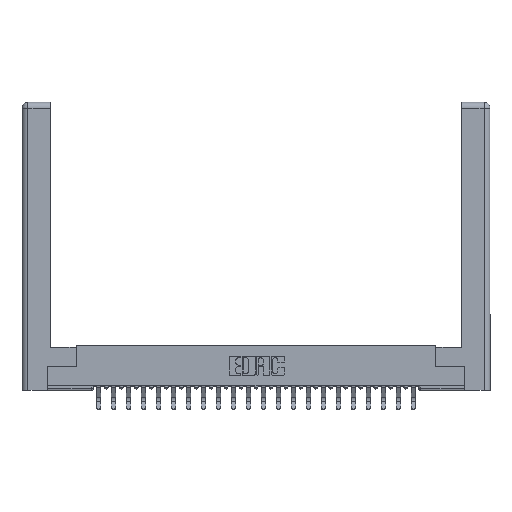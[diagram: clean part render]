
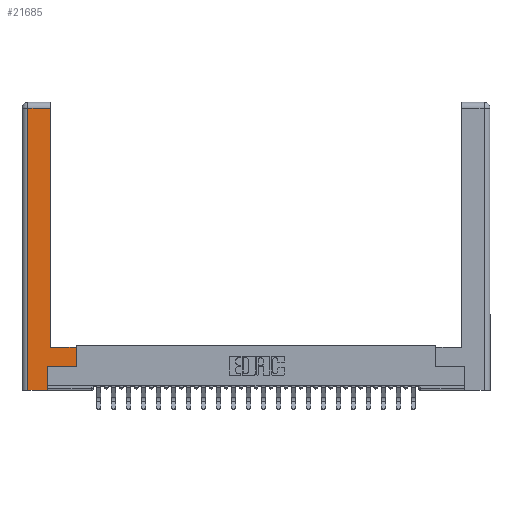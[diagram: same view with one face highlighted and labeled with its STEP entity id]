
A CAD part, top view. The second image highlights one B-rep face of the part: STEP entity #21685.
In plain terms, the highlighted planar face has unit normal (0, 0, 1).
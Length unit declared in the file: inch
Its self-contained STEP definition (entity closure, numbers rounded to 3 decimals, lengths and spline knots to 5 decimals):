
#400 = LINE ( 'NONE', #23113, #10214 ) ;
#420 = CARTESIAN_POINT ( 'NONE',  ( 0.295, 3., 0. ) ) ;
#613 = EDGE_CURVE ( 'NONE', #2396, #14917, #5931, .T. ) ;
#748 = DIRECTION ( 'NONE',  ( -1., 0., 0. ) ) ;
#963 = EDGE_LOOP ( 'NONE', ( #10906, #6641, #12486, #24524, #22520, #22392, #9960, #10470 ) ) ;
#1073 = VECTOR ( 'NONE', #14749, 39.37008 ) ;
#1088 = DIRECTION ( 'NONE',  ( -1., 0., 0. ) ) ;
#1736 = VECTOR ( 'NONE', #748, 39.37008 ) ;
#2396 = VERTEX_POINT ( 'NONE', #5903 ) ;
#2397 = FACE_OUTER_BOUND ( 'NONE', #963, .T. ) ;
#2955 = CARTESIAN_POINT ( 'NONE',  ( 0.0615, 2.94, 0. ) ) ;
#3697 = CARTESIAN_POINT ( 'NONE',  ( 0.265, 0., 0. ) ) ;
#3788 = DIRECTION ( 'NONE',  ( 0., 1., 0. ) ) ;
#4663 = CARTESIAN_POINT ( 'NONE',  ( 0., 0., 0. ) ) ;
#5903 = CARTESIAN_POINT ( 'NONE',  ( 0.295, 0.45, 0. ) ) ;
#5931 = LINE ( 'NONE', #420, #24735 ) ;
#6381 = VERTEX_POINT ( 'NONE', #22027 ) ;
#6532 = DIRECTION ( 'NONE',  ( -1., 0., 0. ) ) ;
#6641 = ORIENTED_EDGE ( 'NONE', *, *, #16748, .T. ) ;
#6659 = CARTESIAN_POINT ( 'NONE',  ( 0.0615, 2.94, 0. ) ) ;
#6730 = CARTESIAN_POINT ( 'NONE',  ( 0.295, 2.94, 0. ) ) ;
#7109 = CARTESIAN_POINT ( 'NONE',  ( 0.565, 0.45, 0. ) ) ;
#7925 = DIRECTION ( 'NONE',  ( 0., -1., 0. ) ) ;
#8385 = AXIS2_PLACEMENT_3D ( 'NONE', #4663, #23725, #6532 ) ;
#8947 = VECTOR ( 'NONE', #18878, 39.37008 ) ;
#9960 = ORIENTED_EDGE ( 'NONE', *, *, #19291, .T. ) ;
#10214 = VECTOR ( 'NONE', #13572, 39.37008 ) ;
#10261 = LINE ( 'NONE', #17926, #1736 ) ;
#10470 = ORIENTED_EDGE ( 'NONE', *, *, #11905, .T. ) ;
#10906 = ORIENTED_EDGE ( 'NONE', *, *, #613, .T. ) ;
#10980 = DIRECTION ( 'NONE',  ( 1., 0., 0. ) ) ;
#11434 = CARTESIAN_POINT ( 'NONE',  ( 0.565, 0.245, 0. ) ) ;
#11905 = EDGE_CURVE ( 'NONE', #16444, #2396, #10261, .T. ) ;
#12083 = VERTEX_POINT ( 'NONE', #3697 ) ;
#12486 = ORIENTED_EDGE ( 'NONE', *, *, #21591, .T. ) ;
#12866 = LINE ( 'NONE', #7109, #1073 ) ;
#13144 = LINE ( 'NONE', #20790, #8947 ) ;
#13359 = EDGE_CURVE ( 'NONE', #16351, #12083, #13144, .T. ) ;
#13572 = DIRECTION ( 'NONE',  ( 0., 1., 0. ) ) ;
#14389 = CARTESIAN_POINT ( 'NONE',  ( 0.565, 0.245, 0. ) ) ;
#14749 = DIRECTION ( 'NONE',  ( 0., 1., 0. ) ) ;
#14767 = VECTOR ( 'NONE', #7925, 39.37008 ) ;
#14917 = VERTEX_POINT ( 'NONE', #6730 ) ;
#16267 = LINE ( 'NONE', #2955, #17851 ) ;
#16351 = VERTEX_POINT ( 'NONE', #16780 ) ;
#16444 = VERTEX_POINT ( 'NONE', #17019 ) ;
#16748 = EDGE_CURVE ( 'NONE', #14917, #24480, #16267, .T. ) ;
#16780 = CARTESIAN_POINT ( 'NONE',  ( 0.0615, 0., 0. ) ) ;
#17019 = CARTESIAN_POINT ( 'NONE',  ( 0.565, 0.45, 0. ) ) ;
#17832 = PLANE ( 'NONE',  #8385 ) ;
#17851 = VECTOR ( 'NONE', #1088, 39.37008 ) ;
#17880 = EDGE_CURVE ( 'NONE', #6381, #24100, #24411, .T. ) ;
#17926 = CARTESIAN_POINT ( 'NONE',  ( 0.295, 0.45, 0. ) ) ;
#18831 = LINE ( 'NONE', #18943, #14767 ) ;
#18878 = DIRECTION ( 'NONE',  ( 1., 0., 0. ) ) ;
#18943 = CARTESIAN_POINT ( 'NONE',  ( 0.0615, 0., 0. ) ) ;
#19291 = EDGE_CURVE ( 'NONE', #24100, #16444, #12866, .T. ) ;
#20790 = CARTESIAN_POINT ( 'NONE',  ( 0.265, 0., 0. ) ) ;
#21591 = EDGE_CURVE ( 'NONE', #24480, #16351, #18831, .T. ) ;
#21685 = ADVANCED_FACE ( 'NONE', ( #2397 ), #17832, .F. ) ;
#22027 = CARTESIAN_POINT ( 'NONE',  ( 0.265, 0.245, 0. ) ) ;
#22392 = ORIENTED_EDGE ( 'NONE', *, *, #17880, .T. ) ;
#22520 = ORIENTED_EDGE ( 'NONE', *, *, #24337, .T. ) ;
#23113 = CARTESIAN_POINT ( 'NONE',  ( 0.265, 0.245, 0. ) ) ;
#23725 = DIRECTION ( 'NONE',  ( 0., 0., -1. ) ) ;
#23834 = VECTOR ( 'NONE', #10980, 39.37008 ) ;
#24100 = VERTEX_POINT ( 'NONE', #11434 ) ;
#24337 = EDGE_CURVE ( 'NONE', #12083, #6381, #400, .T. ) ;
#24411 = LINE ( 'NONE', #14389, #23834 ) ;
#24480 = VERTEX_POINT ( 'NONE', #6659 ) ;
#24524 = ORIENTED_EDGE ( 'NONE', *, *, #13359, .T. ) ;
#24735 = VECTOR ( 'NONE', #3788, 39.37008 ) ;
